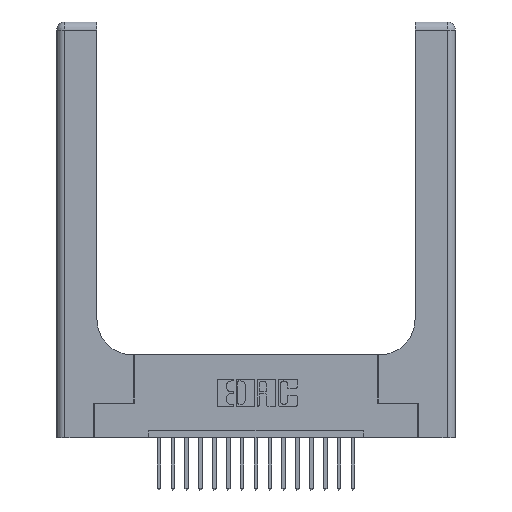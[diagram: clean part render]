
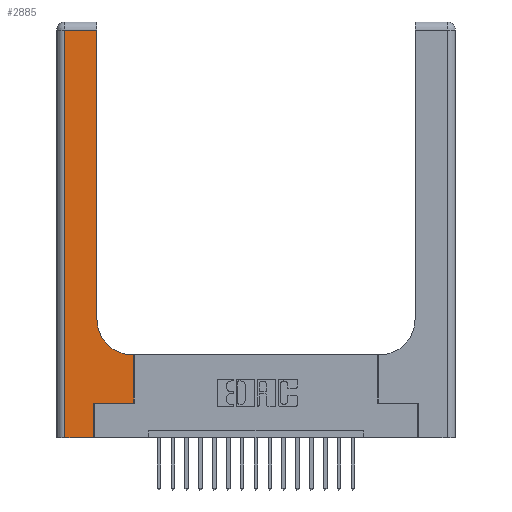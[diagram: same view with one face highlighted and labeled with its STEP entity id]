
A CAD part, top view. The second image highlights one B-rep face of the part: STEP entity #2885.
In plain terms, the highlighted planar face has unit normal (0, 0, 1).
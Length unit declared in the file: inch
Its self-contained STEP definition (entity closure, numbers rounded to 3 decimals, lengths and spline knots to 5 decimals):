
#70 = AXIS2_PLACEMENT_3D ( 'NONE', #8328, #14301, #5187 ) ;
#454 = CARTESIAN_POINT ( 'NONE',  ( 0.2915, 0.85, 0.37 ) ) ;
#846 = LINE ( 'NONE', #2637, #14215 ) ;
#1268 = VECTOR ( 'NONE', #18114, 39.37008 ) ;
#1498 = DIRECTION ( 'NONE',  ( 0., 0., -1. ) ) ;
#1973 = LINE ( 'NONE', #11210, #10479 ) ;
#2350 = CARTESIAN_POINT ( 'NONE',  ( 0.2915, 0.6, 0.37 ) ) ;
#2389 = VERTEX_POINT ( 'NONE', #6897 ) ;
#2568 = LINE ( 'NONE', #20052, #11301 ) ;
#2637 = CARTESIAN_POINT ( 'NONE',  ( 0.5585, 0.25, 0.37 ) ) ;
#2885 = ADVANCED_FACE ( 'NONE', ( #5980 ), #18895, .F. ) ;
#2976 = LINE ( 'NONE', #16368, #1268 ) ;
#3291 = EDGE_CURVE ( 'NONE', #2389, #12686, #5756, .T. ) ;
#3506 = VERTEX_POINT ( 'NONE', #14335 ) ;
#3698 = VERTEX_POINT ( 'NONE', #15451 ) ;
#4092 = EDGE_CURVE ( 'NONE', #14070, #13962, #846, .T. ) ;
#4349 = VERTEX_POINT ( 'NONE', #6299 ) ;
#4959 = ORIENTED_EDGE ( 'NONE', *, *, #6629, .T. ) ;
#5031 = CARTESIAN_POINT ( 'NONE',  ( 0.269, 0., 0.37 ) ) ;
#5187 = DIRECTION ( 'NONE',  ( 1., 0., 0. ) ) ;
#5216 = ORIENTED_EDGE ( 'NONE', *, *, #7861, .T. ) ;
#5756 = CIRCLE ( 'NONE', #70, 0.25 ) ;
#5837 = LINE ( 'NONE', #5031, #13135 ) ;
#5980 = FACE_OUTER_BOUND ( 'NONE', #6436, .T. ) ;
#6215 = EDGE_CURVE ( 'NONE', #15165, #14070, #2976, .T. ) ;
#6299 = CARTESIAN_POINT ( 'NONE',  ( 0.06, 2.94, 0.37 ) ) ;
#6311 = AXIS2_PLACEMENT_3D ( 'NONE', #12496, #1498, #18752 ) ;
#6326 = DIRECTION ( 'NONE',  ( 1., 0., 0. ) ) ;
#6436 = EDGE_LOOP ( 'NONE', ( #18547, #8495, #13734, #4959, #5216, #19162, #9927, #6478, #18968 ) ) ;
#6478 = ORIENTED_EDGE ( 'NONE', *, *, #18556, .T. ) ;
#6533 = VECTOR ( 'NONE', #11864, 39.37008 ) ;
#6629 = EDGE_CURVE ( 'NONE', #3698, #3506, #1973, .T. ) ;
#6853 = VECTOR ( 'NONE', #11695, 39.37008 ) ;
#6894 = VERTEX_POINT ( 'NONE', #16826 ) ;
#6897 = CARTESIAN_POINT ( 'NONE',  ( 0.5415, 0.6, 0.37 ) ) ;
#7036 = LINE ( 'NONE', #11656, #6533 ) ;
#7139 = EDGE_CURVE ( 'NONE', #12686, #6894, #15100, .T. ) ;
#7861 = EDGE_CURVE ( 'NONE', #3506, #15165, #5837, .T. ) ;
#8179 = CARTESIAN_POINT ( 'NONE',  ( 0.2915, 3., 0.37 ) ) ;
#8328 = CARTESIAN_POINT ( 'NONE',  ( 0.5415, 0.85, 0.37 ) ) ;
#8495 = ORIENTED_EDGE ( 'NONE', *, *, #12504, .T. ) ;
#9878 = CARTESIAN_POINT ( 'NONE',  ( 0.269, 0.25, 0.37 ) ) ;
#9927 = ORIENTED_EDGE ( 'NONE', *, *, #4092, .T. ) ;
#10462 = VECTOR ( 'NONE', #11221, 39.37008 ) ;
#10479 = VECTOR ( 'NONE', #6326, 39.37008 ) ;
#11135 = CARTESIAN_POINT ( 'NONE',  ( 0.5585, 0.6, 0.37 ) ) ;
#11210 = CARTESIAN_POINT ( 'NONE',  ( 0., 0., 0.37 ) ) ;
#11221 = DIRECTION ( 'NONE',  ( 0., 1., 0. ) ) ;
#11244 = LINE ( 'NONE', #2350, #6853 ) ;
#11301 = VECTOR ( 'NONE', #12381, 39.37008 ) ;
#11656 = CARTESIAN_POINT ( 'NONE',  ( 0.06, 3., 0.37 ) ) ;
#11695 = DIRECTION ( 'NONE',  ( -1., 0., 0. ) ) ;
#11864 = DIRECTION ( 'NONE',  ( 0., -1., 0. ) ) ;
#12381 = DIRECTION ( 'NONE',  ( -1., 0., 0. ) ) ;
#12496 = CARTESIAN_POINT ( 'NONE',  ( 0., 3., 0.37 ) ) ;
#12504 = EDGE_CURVE ( 'NONE', #6894, #4349, #2568, .T. ) ;
#12686 = VERTEX_POINT ( 'NONE', #454 ) ;
#13135 = VECTOR ( 'NONE', #16516, 39.37008 ) ;
#13734 = ORIENTED_EDGE ( 'NONE', *, *, #14720, .T. ) ;
#13962 = VERTEX_POINT ( 'NONE', #11135 ) ;
#14070 = VERTEX_POINT ( 'NONE', #15717 ) ;
#14215 = VECTOR ( 'NONE', #18324, 39.37008 ) ;
#14301 = DIRECTION ( 'NONE',  ( 0., 0., -1. ) ) ;
#14335 = CARTESIAN_POINT ( 'NONE',  ( 0.269, 0., 0.37 ) ) ;
#14720 = EDGE_CURVE ( 'NONE', #4349, #3698, #7036, .T. ) ;
#15100 = LINE ( 'NONE', #8179, #10462 ) ;
#15165 = VERTEX_POINT ( 'NONE', #9878 ) ;
#15451 = CARTESIAN_POINT ( 'NONE',  ( 0.06, 0., 0.37 ) ) ;
#15717 = CARTESIAN_POINT ( 'NONE',  ( 0.5585, 0.25, 0.37 ) ) ;
#16368 = CARTESIAN_POINT ( 'NONE',  ( 0.269, 0.25, 0.37 ) ) ;
#16516 = DIRECTION ( 'NONE',  ( 0., 1., 0. ) ) ;
#16826 = CARTESIAN_POINT ( 'NONE',  ( 0.2915, 2.94, 0.37 ) ) ;
#18114 = DIRECTION ( 'NONE',  ( 1., 0., 0. ) ) ;
#18324 = DIRECTION ( 'NONE',  ( 0., 1., 0. ) ) ;
#18547 = ORIENTED_EDGE ( 'NONE', *, *, #7139, .T. ) ;
#18556 = EDGE_CURVE ( 'NONE', #13962, #2389, #11244, .T. ) ;
#18752 = DIRECTION ( 'NONE',  ( -1., 0., 0. ) ) ;
#18895 = PLANE ( 'NONE',  #6311 ) ;
#18968 = ORIENTED_EDGE ( 'NONE', *, *, #3291, .T. ) ;
#19162 = ORIENTED_EDGE ( 'NONE', *, *, #6215, .T. ) ;
#20052 = CARTESIAN_POINT ( 'NONE',  ( 0., 2.94, 0.37 ) ) ;
